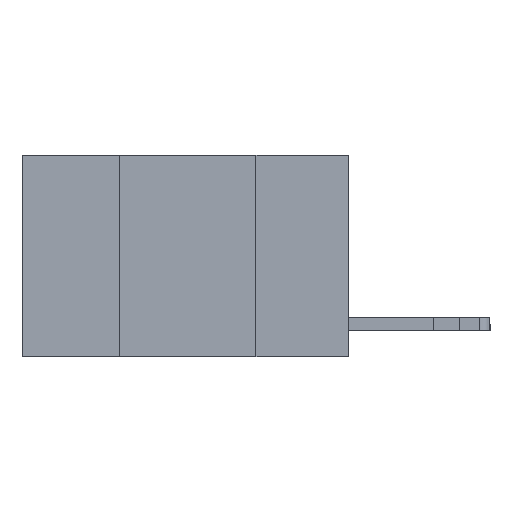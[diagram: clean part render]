
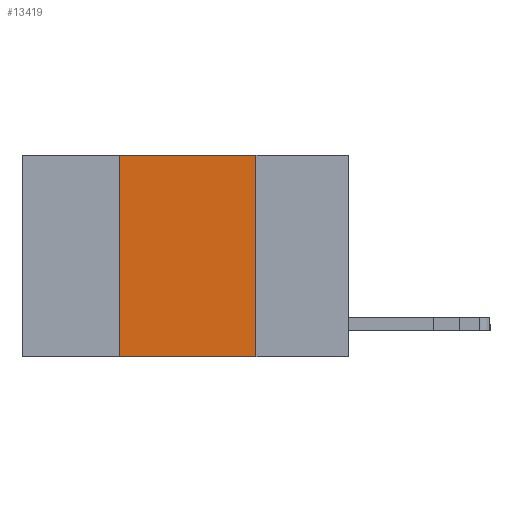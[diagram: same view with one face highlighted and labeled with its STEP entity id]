
A CAD part, left-side view. The second image highlights one B-rep face of the part: STEP entity #13419.
In plain terms, the highlighted planar face has unit normal (-1, 0, 0).
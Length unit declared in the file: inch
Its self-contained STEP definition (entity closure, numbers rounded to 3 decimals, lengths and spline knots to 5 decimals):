
#495 = VECTOR ( 'NONE', #4568, 39.37008 ) ;
#920 = FACE_OUTER_BOUND ( 'NONE', #1359, .T. ) ;
#1304 = ORIENTED_EDGE ( 'NONE', *, *, #6268, .T. ) ;
#1359 = EDGE_LOOP ( 'NONE', ( #9453, #10946, #12050, #1304 ) ) ;
#2225 = DIRECTION ( 'NONE',  ( 1., 0., 0. ) ) ;
#2467 = EDGE_CURVE ( 'NONE', #11251, #5627, #10416, .T. ) ;
#2539 = LINE ( 'NONE', #6265, #5678 ) ;
#2983 = CARTESIAN_POINT ( 'NONE',  ( 0., 0.6, 0. ) ) ;
#3427 = PLANE ( 'NONE',  #8972 ) ;
#3701 = EDGE_CURVE ( 'NONE', #5627, #7289, #7632, .T. ) ;
#3836 = DIRECTION ( 'NONE',  ( 0., -1., 0. ) ) ;
#4243 = VECTOR ( 'NONE', #13041, 39.37008 ) ;
#4411 = CARTESIAN_POINT ( 'NONE',  ( 0., 0.42, 0. ) ) ;
#4568 = DIRECTION ( 'NONE',  ( 0., 0., 1. ) ) ;
#4816 = VECTOR ( 'NONE', #12732, 39.37008 ) ;
#5627 = VERTEX_POINT ( 'NONE', #14649 ) ;
#5678 = VECTOR ( 'NONE', #3836, 39.37008 ) ;
#6265 = CARTESIAN_POINT ( 'NONE',  ( 0., 0.6, -0.37 ) ) ;
#6268 = EDGE_CURVE ( 'NONE', #13138, #7289, #2539, .T. ) ;
#7094 = DIRECTION ( 'NONE',  ( 0., 0., -1. ) ) ;
#7162 = CARTESIAN_POINT ( 'NONE',  ( 0., 0.17, -0.37 ) ) ;
#7289 = VERTEX_POINT ( 'NONE', #7162 ) ;
#7632 = LINE ( 'NONE', #12654, #4816 ) ;
#8972 = AXIS2_PLACEMENT_3D ( 'NONE', #12442, #2225, #7094 ) ;
#9453 = ORIENTED_EDGE ( 'NONE', *, *, #3701, .F. ) ;
#10416 = LINE ( 'NONE', #2983, #4243 ) ;
#10500 = CARTESIAN_POINT ( 'NONE',  ( 0., 0.42, 0. ) ) ;
#10946 = ORIENTED_EDGE ( 'NONE', *, *, #2467, .F. ) ;
#11251 = VERTEX_POINT ( 'NONE', #10500 ) ;
#11383 = CARTESIAN_POINT ( 'NONE',  ( 0., 0.42, -0.37 ) ) ;
#12050 = ORIENTED_EDGE ( 'NONE', *, *, #15094, .F. ) ;
#12442 = CARTESIAN_POINT ( 'NONE',  ( 0., 0.6, 0. ) ) ;
#12654 = CARTESIAN_POINT ( 'NONE',  ( 0., 0.17, 0. ) ) ;
#12732 = DIRECTION ( 'NONE',  ( 0., 0., -1. ) ) ;
#13041 = DIRECTION ( 'NONE',  ( 0., -1., 0. ) ) ;
#13138 = VERTEX_POINT ( 'NONE', #11383 ) ;
#13419 = ADVANCED_FACE ( 'NONE', ( #920 ), #3427, .F. ) ;
#14649 = CARTESIAN_POINT ( 'NONE',  ( 0., 0.17, 0. ) ) ;
#15094 = EDGE_CURVE ( 'NONE', #13138, #11251, #15605, .T. ) ;
#15605 = LINE ( 'NONE', #4411, #495 ) ;
